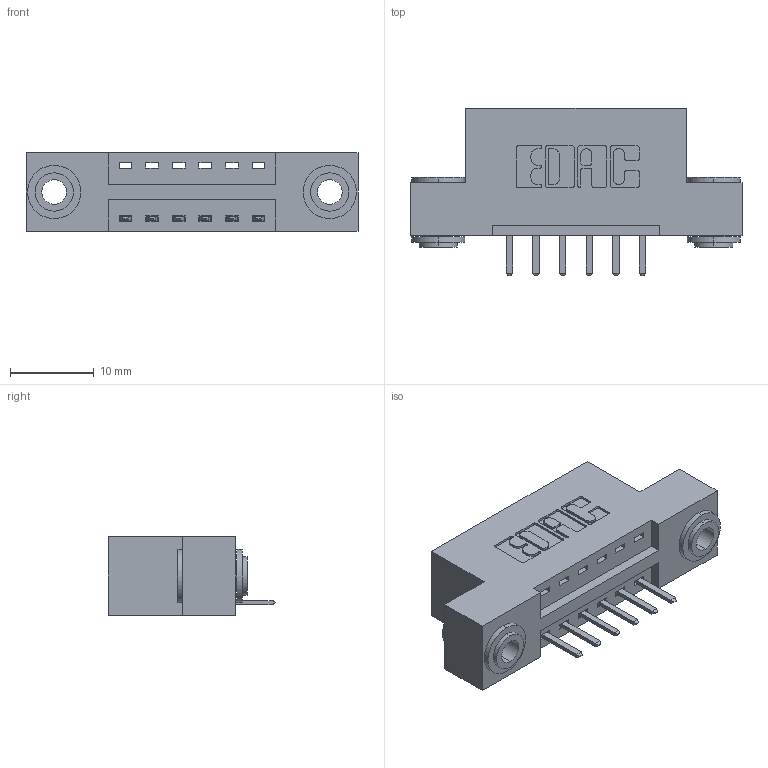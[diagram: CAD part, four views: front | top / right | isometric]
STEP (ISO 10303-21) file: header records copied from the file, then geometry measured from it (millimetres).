
FILE_DESCRIPTION (( 'STEP AP203' ), '1' );
FILE_NAME ('346-006-520-103.STEP', '2022-05-04T18:21:58', ( '' ), ( '' ), 'SwSTEP 2.0', 'SolidWorks 2020', '' );
FILE_SCHEMA (( 'CONFIG_CONTROL_DESIGN' ));
Length unit declared in the file: inch
Products named in the file (4): 346 Part_Flush Mounting Lugs - 0.156 Dia-TH; 346-006-520-103; 345-250-002_345-250-002-102; 345-292-001_345-293-120
Assembly tree (9 placements, depth 2):
  346-006-520-103
    346 Part_Flush Mounting Lugs - 0.156 Dia-TH
    345-292-001_345-293-120  x6
    345-250-002_345-250-002-102  x2
Bounding box: 39.62 x 20.02 x 9.4 mm (x, y, z)
Volume: 3528.9 mm3; surface area: 4216 mm2
Topology: 9 solids, 9 shells, 546 faces, 1545 edges, 1010 vertices
Faces by surface type: plane 352, cylinder 186, cone 8
Entity records: 9750 total; most frequent: CARTESIAN_POINT 1675, ORIENTED_EDGE 1594, DIRECTION 1539, EDGE_CURVE 797, VECTOR 613, LINE 613, VERTEX_POINT 526, AXIS2_PLACEMENT_3D 463
